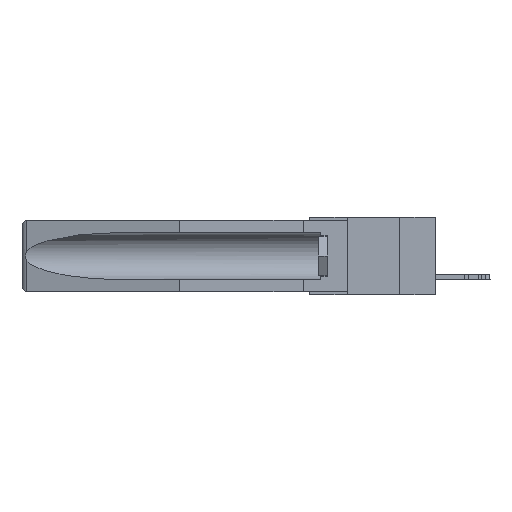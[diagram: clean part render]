
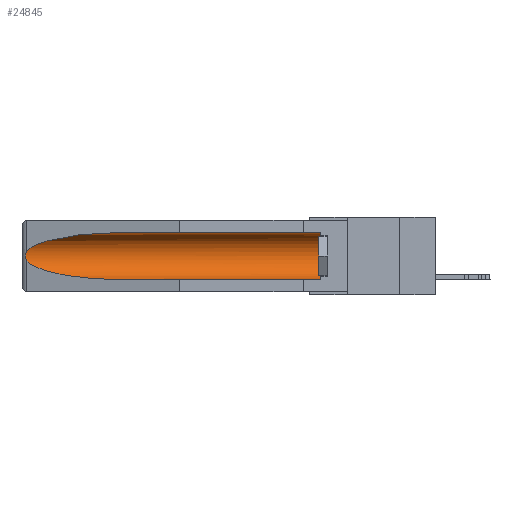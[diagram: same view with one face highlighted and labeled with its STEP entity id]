
A CAD part, left-side view. The second image highlights one B-rep face of the part: STEP entity #24845.
In plain terms, the highlighted cylindrical face has radius 2.857 mm (diameter 5.715 mm), a partial arc.
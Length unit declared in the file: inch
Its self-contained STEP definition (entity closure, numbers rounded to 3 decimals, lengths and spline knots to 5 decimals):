
#346 = AXIS2_PLACEMENT_3D ( 'NONE', #17070, #14947, #915 ) ;
#411 = B_SPLINE_CURVE_WITH_KNOTS ( 'NONE', 3,
 ( #11275, #20853, #27466, #23100, #11594, #23199, #8875, #8979, #21227, #25438 ),
 .UNSPECIFIED., .F., .F.,
 ( 4, 2, 2, 2, 4 ),
 ( 0., 0.00029, 0.00058, 0.00087, 0.00117 ),
 .UNSPECIFIED. ) ;
#915 = DIRECTION ( 'NONE',  ( 0., 0., 1. ) ) ;
#1469 = CARTESIAN_POINT ( 'NONE',  ( 0.26537, 1.52718, -0.14972 ) ) ;
#1734 = CARTESIAN_POINT ( 'NONE',  ( 0.26537, 1.52718, -0.19328 ) ) ;
#1736 = LINE ( 'NONE', #21871, #4256 ) ;
#2067 = CARTESIAN_POINT ( 'NONE',  ( 0.155, 0.126, -0.1715 ) ) ;
#2171 = DIRECTION ( 'NONE',  ( 0., 0., 1. ) ) ;
#3399 = EDGE_CURVE ( 'NONE', #28555, #9708, #12322, .T. ) ;
#3409 = CARTESIAN_POINT ( 'NONE',  ( 0.155, -0.30754, -0.059 ) ) ;
#3475 = ORIENTED_EDGE ( 'NONE', *, *, #25060, .T. ) ;
#4256 = VECTOR ( 'NONE', #19423, 39.37008 ) ;
#4963 = EDGE_CURVE ( 'NONE', #9708, #24760, #20569, .T. ) ;
#5194 = CARTESIAN_POINT ( 'NONE',  ( 0.26537, 1.52718, -0.14972 ) ) ;
#6208 = VERTEX_POINT ( 'NONE', #12301 ) ;
#6219 = CARTESIAN_POINT ( 'NONE',  ( 0.21114, 1.30732, -0.059 ) ) ;
#7991 = VERTEX_POINT ( 'NONE', #1734 ) ;
#8001 =( BOUNDED_CURVE ( )  B_SPLINE_CURVE ( 3, ( #13019, #24309, #24506, #22077 ),
 .UNSPECIFIED., .F., .F. ) 
 B_SPLINE_CURVE_WITH_KNOTS ( ( 4, 4 ),
 ( 0.1948, 1.5708 ),
 .UNSPECIFIED. ) 
 CURVE ( )  GEOMETRIC_REPRESENTATION_ITEM ( )  RATIONAL_B_SPLINE_CURVE ( ( 1., 0.848, 0.848, 1. ) ) 
 REPRESENTATION_ITEM ( '' )  );
#8875 = CARTESIAN_POINT ( 'NONE',  ( 0.2673, 1.53269, -0.17917 ) ) ;
#8979 = CARTESIAN_POINT ( 'NONE',  ( 0.26655, 1.53094, -0.18657 ) ) ;
#9628 = CARTESIAN_POINT ( 'NONE',  ( 0.155, 0.126, -0.059 ) ) ;
#9675 = VECTOR ( 'NONE', #21740, 39.37008 ) ;
#9708 = VERTEX_POINT ( 'NONE', #9628 ) ;
#11150 = EDGE_CURVE ( 'NONE', #28555, #6208, #1736, .T. ) ;
#11275 = CARTESIAN_POINT ( 'NONE',  ( 0.26537, 1.52718, -0.14972 ) ) ;
#11594 = CARTESIAN_POINT ( 'NONE',  ( 0.2675, 1.53308, -0.16763 ) ) ;
#12132 = CARTESIAN_POINT ( 'NONE',  ( 0.155, 1.07973, -0.059 ) ) ;
#12301 = CARTESIAN_POINT ( 'NONE',  ( 0.155, 1.07973, -0.284 ) ) ;
#12322 = CIRCLE ( 'NONE', #22487, 0.1125 ) ;
#13019 = CARTESIAN_POINT ( 'NONE',  ( 0.26537, 1.52718, -0.19328 ) ) ;
#13082 = FACE_OUTER_BOUND ( 'NONE', #19990, .T. ) ;
#13192 = ORIENTED_EDGE ( 'NONE', *, *, #20532, .T. ) ;
#14947 = DIRECTION ( 'NONE',  ( 0., 1., 0. ) ) ;
#15319 = ORIENTED_EDGE ( 'NONE', *, *, #4963, .T. ) ;
#15407 = CARTESIAN_POINT ( 'NONE',  ( 0.155, 1.07973, -0.059 ) ) ;
#16228 = ORIENTED_EDGE ( 'NONE', *, *, #21440, .T. ) ;
#17070 = CARTESIAN_POINT ( 'NONE',  ( 0.155, -0.30754, -0.1715 ) ) ;
#17414 = CYLINDRICAL_SURFACE ( 'NONE', #346, 0.1125 ) ;
#19141 = ORIENTED_EDGE ( 'NONE', *, *, #3399, .T. ) ;
#19423 = DIRECTION ( 'NONE',  ( 0., 1., 0. ) ) ;
#19990 = EDGE_LOOP ( 'NONE', ( #16228, #13192, #3475, #27569, #19141, #15319 ) ) ;
#20532 = EDGE_CURVE ( 'NONE', #21837, #7991, #411, .T. ) ;
#20569 = LINE ( 'NONE', #3409, #9675 ) ;
#20595 = DIRECTION ( 'NONE',  ( 0., -1., 0. ) ) ;
#20853 = CARTESIAN_POINT ( 'NONE',  ( 0.26597, 1.52961, -0.15275 ) ) ;
#21227 = CARTESIAN_POINT ( 'NONE',  ( 0.26597, 1.5296, -0.19026 ) ) ;
#21440 = EDGE_CURVE ( 'NONE', #24760, #21837, #27343, .T. ) ;
#21740 = DIRECTION ( 'NONE',  ( 0., 1., 0. ) ) ;
#21837 = VERTEX_POINT ( 'NONE', #5194 ) ;
#21871 = CARTESIAN_POINT ( 'NONE',  ( 0.155, -0.30754, -0.284 ) ) ;
#22077 = CARTESIAN_POINT ( 'NONE',  ( 0.155, 1.07973, -0.284 ) ) ;
#22131 = CARTESIAN_POINT ( 'NONE',  ( 0.25451, 1.48313, -0.09465 ) ) ;
#22487 = AXIS2_PLACEMENT_3D ( 'NONE', #2067, #20595, #2171 ) ;
#23100 = CARTESIAN_POINT ( 'NONE',  ( 0.2673, 1.5327, -0.16383 ) ) ;
#23199 = CARTESIAN_POINT ( 'NONE',  ( 0.2675, 1.53308, -0.17534 ) ) ;
#23375 = CARTESIAN_POINT ( 'NONE',  ( 0.155, 0.126, -0.284 ) ) ;
#24309 = CARTESIAN_POINT ( 'NONE',  ( 0.25451, 1.48313, -0.24835 ) ) ;
#24506 = CARTESIAN_POINT ( 'NONE',  ( 0.21114, 1.30732, -0.284 ) ) ;
#24760 = VERTEX_POINT ( 'NONE', #12132 ) ;
#24845 = ADVANCED_FACE ( 'NONE', ( #13082 ), #17414, .F. ) ;
#25060 = EDGE_CURVE ( 'NONE', #7991, #6208, #8001, .T. ) ;
#25438 = CARTESIAN_POINT ( 'NONE',  ( 0.26537, 1.52718, -0.19328 ) ) ;
#27343 =( BOUNDED_CURVE ( )  B_SPLINE_CURVE ( 3, ( #15407, #6219, #22131, #1469 ),
 .UNSPECIFIED., .F., .F. ) 
 B_SPLINE_CURVE_WITH_KNOTS ( ( 4, 4 ),
 ( 4.71239, 6.08839 ),
 .UNSPECIFIED. ) 
 CURVE ( )  GEOMETRIC_REPRESENTATION_ITEM ( )  RATIONAL_B_SPLINE_CURVE ( ( 1., 0.848, 0.848, 1. ) ) 
 REPRESENTATION_ITEM ( '' )  );
#27466 = CARTESIAN_POINT ( 'NONE',  ( 0.26654, 1.53092, -0.15636 ) ) ;
#27569 = ORIENTED_EDGE ( 'NONE', *, *, #11150, .F. ) ;
#28555 = VERTEX_POINT ( 'NONE', #23375 ) ;
